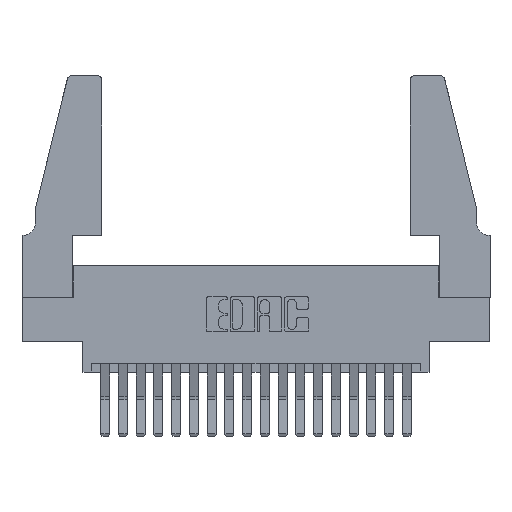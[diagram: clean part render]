
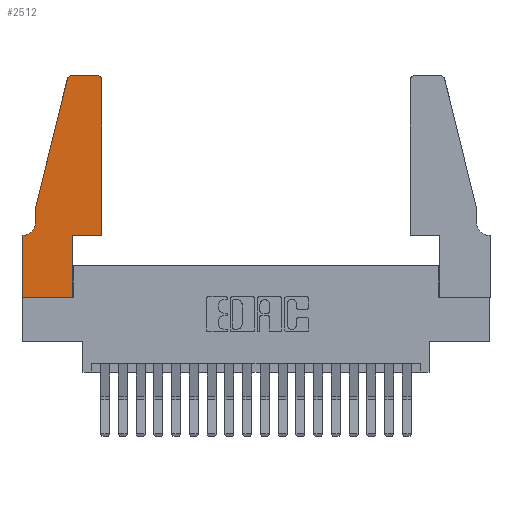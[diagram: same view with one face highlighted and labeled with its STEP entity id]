
A CAD part, top view. The second image highlights one B-rep face of the part: STEP entity #2512.
In plain terms, the highlighted planar face has unit normal (0, 0, 1).
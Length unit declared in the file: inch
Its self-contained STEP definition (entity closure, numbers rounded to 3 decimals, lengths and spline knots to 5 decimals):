
#29 = DIRECTION ( 'NONE',  ( 0., 0., -1. ) ) ;
#141 = VERTEX_POINT ( 'NONE', #16963 ) ;
#155 = VERTEX_POINT ( 'NONE', #3302 ) ;
#547 = DIRECTION ( 'NONE',  ( 0., -1., 0. ) ) ;
#619 = CARTESIAN_POINT ( 'NONE',  ( 0.0755, 0.5, 0.37 ) ) ;
#733 = VECTOR ( 'NONE', #547, 39.37008 ) ;
#1032 = VERTEX_POINT ( 'NONE', #19061 ) ;
#1466 = VECTOR ( 'NONE', #6892, 39.37008 ) ;
#1496 = VERTEX_POINT ( 'NONE', #15325 ) ;
#1508 = CARTESIAN_POINT ( 'NONE',  ( 0.0755, 0.5, 0.37 ) ) ;
#2213 = LINE ( 'NONE', #19478, #4142 ) ;
#2217 = CIRCLE ( 'NONE', #19671, 0.07 ) ;
#2428 = EDGE_CURVE ( 'NONE', #5947, #19056, #18738, .T. ) ;
#2512 = ADVANCED_FACE ( 'NONE', ( #7051 ), #5105, .T. ) ;
#2960 = CARTESIAN_POINT ( 'NONE',  ( 0., 0.35, 0.37 ) ) ;
#3112 = EDGE_CURVE ( 'NONE', #13929, #4787, #13457, .T. ) ;
#3302 = CARTESIAN_POINT ( 'NONE',  ( 0.2865, 0.35, 0.37 ) ) ;
#3523 = EDGE_CURVE ( 'NONE', #1032, #13929, #2217, .T. ) ;
#3596 = DIRECTION ( 'NONE',  ( 1., 0., 0. ) ) ;
#3897 = CARTESIAN_POINT ( 'NONE',  ( 0.4205, 1.25, 0.37 ) ) ;
#3901 = ORIENTED_EDGE ( 'NONE', *, *, #12313, .T. ) ;
#4061 = CARTESIAN_POINT ( 'NONE',  ( 0.284, 1.22, 0.37 ) ) ;
#4106 = AXIS2_PLACEMENT_3D ( 'NONE', #9236, #7847, #13902 ) ;
#4142 = VECTOR ( 'NONE', #14981, 39.37008 ) ;
#4247 = ORIENTED_EDGE ( 'NONE', *, *, #3112, .T. ) ;
#4304 = CARTESIAN_POINT ( 'NONE',  ( 0.4505, 0.35, 0.37 ) ) ;
#4447 = VECTOR ( 'NONE', #6642, 39.37008 ) ;
#4720 = CARTESIAN_POINT ( 'NONE',  ( 0.284, 1.25, 0.37 ) ) ;
#4787 = VERTEX_POINT ( 'NONE', #2960 ) ;
#5105 = PLANE ( 'NONE',  #13642 ) ;
#5113 = CARTESIAN_POINT ( 'NONE',  ( 0.0755, 0.5, 0.37 ) ) ;
#5257 = LINE ( 'NONE', #9269, #733 ) ;
#5504 = DIRECTION ( 'NONE',  ( 0., 0., 1. ) ) ;
#5947 = VERTEX_POINT ( 'NONE', #15152 ) ;
#6056 = VECTOR ( 'NONE', #18047, 39.37008 ) ;
#6081 = VECTOR ( 'NONE', #6087, 39.37008 ) ;
#6087 = DIRECTION ( 'NONE',  ( 0., 1., 0. ) ) ;
#6448 = CARTESIAN_POINT ( 'NONE',  ( 0., 0., 0.37 ) ) ;
#6642 = DIRECTION ( 'NONE',  ( -1., 0., 0. ) ) ;
#6714 = CARTESIAN_POINT ( 'NONE',  ( 0.0055, 0.35, 0.37 ) ) ;
#6771 = VECTOR ( 'NONE', #16566, 39.37008 ) ;
#6892 = DIRECTION ( 'NONE',  ( 0., -1., 0. ) ) ;
#6934 = ORIENTED_EDGE ( 'NONE', *, *, #11393, .T. ) ;
#6990 = AXIS2_PLACEMENT_3D ( 'NONE', #4061, #5504, #11595 ) ;
#7051 = FACE_OUTER_BOUND ( 'NONE', #16018, .T. ) ;
#7304 = CARTESIAN_POINT ( 'NONE',  ( 0.2865, 0.35, 0.37 ) ) ;
#7847 = DIRECTION ( 'NONE',  ( 0., 0., 1. ) ) ;
#8201 = CARTESIAN_POINT ( 'NONE',  ( 0., 0.35, 0.37 ) ) ;
#8647 = ORIENTED_EDGE ( 'NONE', *, *, #16007, .T. ) ;
#8776 = CARTESIAN_POINT ( 'NONE',  ( 0.25487, 1.22718, 0.37 ) ) ;
#8830 = CARTESIAN_POINT ( 'NONE',  ( 0.0755, 0.35, 0.37 ) ) ;
#9036 = DIRECTION ( 'NONE',  ( -0.239, -0.971, 0. ) ) ;
#9187 = ORIENTED_EDGE ( 'NONE', *, *, #9368, .T. ) ;
#9236 = CARTESIAN_POINT ( 'NONE',  ( 0.4205, 1.22, 0.37 ) ) ;
#9269 = CARTESIAN_POINT ( 'NONE',  ( 0., 0., 0.37 ) ) ;
#9368 = EDGE_CURVE ( 'NONE', #19056, #155, #10129, .T. ) ;
#9905 = EDGE_CURVE ( 'NONE', #141, #1496, #11071, .T. ) ;
#9925 = ORIENTED_EDGE ( 'NONE', *, *, #16634, .T. ) ;
#9948 = ORIENTED_EDGE ( 'NONE', *, *, #17212, .T. ) ;
#10030 = VERTEX_POINT ( 'NONE', #4720 ) ;
#10129 = LINE ( 'NONE', #7304, #6081 ) ;
#10346 = ORIENTED_EDGE ( 'NONE', *, *, #11727, .T. ) ;
#10458 = VERTEX_POINT ( 'NONE', #5113 ) ;
#10522 = LINE ( 'NONE', #619, #1466 ) ;
#10982 = DIRECTION ( 'NONE',  ( 1., 0., 0. ) ) ;
#11071 = LINE ( 'NONE', #4304, #6771 ) ;
#11144 = VERTEX_POINT ( 'NONE', #8776 ) ;
#11393 = EDGE_CURVE ( 'NONE', #10458, #1032, #10522, .T. ) ;
#11595 = DIRECTION ( 'NONE',  ( 1., 0., 0. ) ) ;
#11635 = ORIENTED_EDGE ( 'NONE', *, *, #2428, .T. ) ;
#11727 = EDGE_CURVE ( 'NONE', #4787, #5947, #5257, .T. ) ;
#12073 = LINE ( 'NONE', #14036, #4447 ) ;
#12158 = DIRECTION ( 'NONE',  ( -1., 0., 0. ) ) ;
#12266 = CIRCLE ( 'NONE', #4106, 0.03 ) ;
#12313 = EDGE_CURVE ( 'NONE', #10030, #11144, #15973, .T. ) ;
#13457 = LINE ( 'NONE', #8830, #6056 ) ;
#13642 = AXIS2_PLACEMENT_3D ( 'NONE', #8201, #18849, #10982 ) ;
#13902 = DIRECTION ( 'NONE',  ( 1., 0., 0. ) ) ;
#13929 = VERTEX_POINT ( 'NONE', #6714 ) ;
#13930 = LINE ( 'NONE', #1508, #15582 ) ;
#14036 = CARTESIAN_POINT ( 'NONE',  ( 0.2605, 1.25, 0.37 ) ) ;
#14097 = ORIENTED_EDGE ( 'NONE', *, *, #9905, .T. ) ;
#14414 = VECTOR ( 'NONE', #3596, 39.37008 ) ;
#14820 = EDGE_CURVE ( 'NONE', #19392, #10030, #12073, .T. ) ;
#14981 = DIRECTION ( 'NONE',  ( 1., 0., 0. ) ) ;
#15152 = CARTESIAN_POINT ( 'NONE',  ( 0., 0., 0.37 ) ) ;
#15325 = CARTESIAN_POINT ( 'NONE',  ( 0.4505, 1.22, 0.37 ) ) ;
#15329 = CARTESIAN_POINT ( 'NONE',  ( 0.0055, 0.42, 0.37 ) ) ;
#15582 = VECTOR ( 'NONE', #9036, 39.37008 ) ;
#15973 = CIRCLE ( 'NONE', #6990, 0.03 ) ;
#16007 = EDGE_CURVE ( 'NONE', #1496, #19392, #12266, .T. ) ;
#16018 = EDGE_LOOP ( 'NONE', ( #16307, #3901, #9925, #6934, #16310, #4247, #10346, #11635, #9187, #9948, #14097, #8647 ) ) ;
#16307 = ORIENTED_EDGE ( 'NONE', *, *, #14820, .T. ) ;
#16310 = ORIENTED_EDGE ( 'NONE', *, *, #3523, .T. ) ;
#16566 = DIRECTION ( 'NONE',  ( 0., 1., 0. ) ) ;
#16634 = EDGE_CURVE ( 'NONE', #11144, #10458, #13930, .T. ) ;
#16963 = CARTESIAN_POINT ( 'NONE',  ( 0.4505, 0.35, 0.37 ) ) ;
#17212 = EDGE_CURVE ( 'NONE', #155, #141, #2213, .T. ) ;
#18047 = DIRECTION ( 'NONE',  ( -1., 0., 0. ) ) ;
#18738 = LINE ( 'NONE', #6448, #14414 ) ;
#18849 = DIRECTION ( 'NONE',  ( 0., 0., 1. ) ) ;
#19056 = VERTEX_POINT ( 'NONE', #19340 ) ;
#19061 = CARTESIAN_POINT ( 'NONE',  ( 0.0755, 0.42, 0.37 ) ) ;
#19340 = CARTESIAN_POINT ( 'NONE',  ( 0.2865, 0., 0.37 ) ) ;
#19392 = VERTEX_POINT ( 'NONE', #3897 ) ;
#19478 = CARTESIAN_POINT ( 'NONE',  ( 0.4505, 0.35, 0.37 ) ) ;
#19671 = AXIS2_PLACEMENT_3D ( 'NONE', #15329, #29, #12158 ) ;
